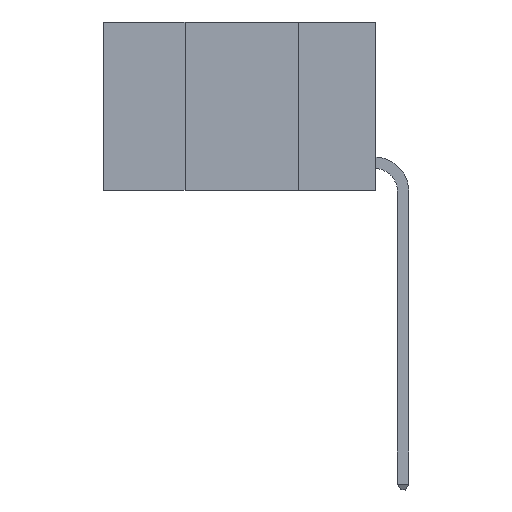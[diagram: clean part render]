
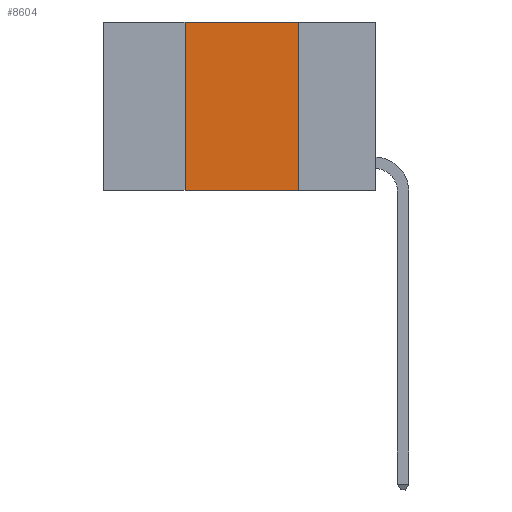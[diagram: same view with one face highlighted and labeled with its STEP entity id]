
A CAD part, left-side view. The second image highlights one B-rep face of the part: STEP entity #8604.
In plain terms, the highlighted planar face has unit normal (-1, 0, 0).
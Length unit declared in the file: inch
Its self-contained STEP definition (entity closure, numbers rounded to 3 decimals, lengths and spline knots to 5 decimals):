
#100 = CARTESIAN_POINT ( 'NONE',  ( 0., 0.42, 0. ) ) ;
#314 = LINE ( 'NONE', #949, #7541 ) ;
#468 = CARTESIAN_POINT ( 'NONE',  ( 0., 0.17, 0. ) ) ;
#470 = VECTOR ( 'NONE', #7559, 39.37008 ) ;
#949 = CARTESIAN_POINT ( 'NONE',  ( 0., 0.6, -0.37 ) ) ;
#968 = ORIENTED_EDGE ( 'NONE', *, *, #4475, .T. ) ;
#1132 = ORIENTED_EDGE ( 'NONE', *, *, #2568, .F. ) ;
#1362 = ORIENTED_EDGE ( 'NONE', *, *, #1393, .F. ) ;
#1393 = EDGE_CURVE ( 'NONE', #7967, #5735, #3134, .T. ) ;
#1404 = VECTOR ( 'NONE', #2551, 39.37008 ) ;
#2322 = AXIS2_PLACEMENT_3D ( 'NONE', #5081, #7886, #3721 ) ;
#2335 = VERTEX_POINT ( 'NONE', #6111 ) ;
#2551 = DIRECTION ( 'NONE',  ( 0., 0., -1. ) ) ;
#2568 = EDGE_CURVE ( 'NONE', #4439, #7967, #3109, .T. ) ;
#3023 = PLANE ( 'NONE',  #2322 ) ;
#3109 = LINE ( 'NONE', #6018, #4965 ) ;
#3134 = LINE ( 'NONE', #468, #1404 ) ;
#3721 = DIRECTION ( 'NONE',  ( 0., 0., -1. ) ) ;
#3724 = EDGE_CURVE ( 'NONE', #2335, #4439, #6286, .T. ) ;
#4439 = VERTEX_POINT ( 'NONE', #100 ) ;
#4475 = EDGE_CURVE ( 'NONE', #2335, #5735, #314, .T. ) ;
#4591 = DIRECTION ( 'NONE',  ( 0., -1., 0. ) ) ;
#4965 = VECTOR ( 'NONE', #6015, 39.37008 ) ;
#5081 = CARTESIAN_POINT ( 'NONE',  ( 0., 0.6, 0. ) ) ;
#5735 = VERTEX_POINT ( 'NONE', #8033 ) ;
#5869 = EDGE_LOOP ( 'NONE', ( #1362, #1132, #7961, #968 ) ) ;
#6015 = DIRECTION ( 'NONE',  ( 0., -1., 0. ) ) ;
#6018 = CARTESIAN_POINT ( 'NONE',  ( 0., 0.6, 0. ) ) ;
#6111 = CARTESIAN_POINT ( 'NONE',  ( 0., 0.42, -0.37 ) ) ;
#6286 = LINE ( 'NONE', #7432, #470 ) ;
#6375 = CARTESIAN_POINT ( 'NONE',  ( 0., 0.17, 0. ) ) ;
#6639 = FACE_OUTER_BOUND ( 'NONE', #5869, .T. ) ;
#7432 = CARTESIAN_POINT ( 'NONE',  ( 0., 0.42, 0. ) ) ;
#7541 = VECTOR ( 'NONE', #4591, 39.37008 ) ;
#7559 = DIRECTION ( 'NONE',  ( 0., 0., 1. ) ) ;
#7886 = DIRECTION ( 'NONE',  ( 1., 0., 0. ) ) ;
#7961 = ORIENTED_EDGE ( 'NONE', *, *, #3724, .F. ) ;
#7967 = VERTEX_POINT ( 'NONE', #6375 ) ;
#8033 = CARTESIAN_POINT ( 'NONE',  ( 0., 0.17, -0.37 ) ) ;
#8604 = ADVANCED_FACE ( 'NONE', ( #6639 ), #3023, .F. ) ;
